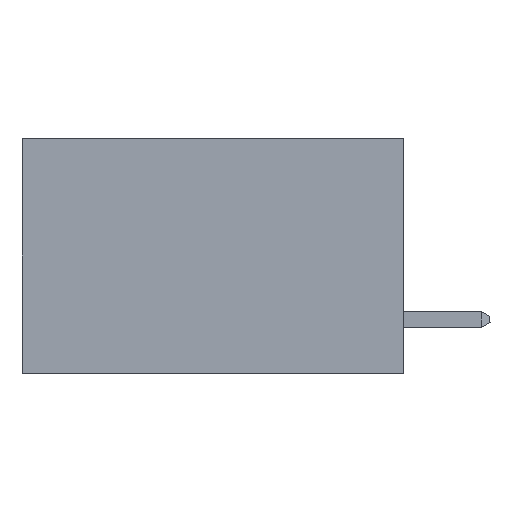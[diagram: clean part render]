
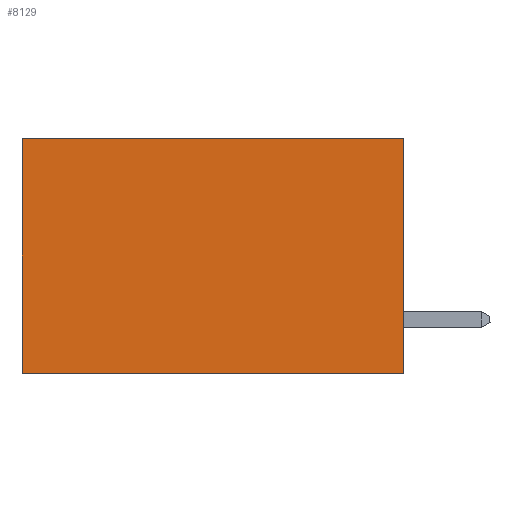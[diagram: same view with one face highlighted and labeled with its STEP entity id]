
A CAD part, left-side view. The second image highlights one B-rep face of the part: STEP entity #8129.
In plain terms, the highlighted planar face has unit normal (-1, 0, 0).
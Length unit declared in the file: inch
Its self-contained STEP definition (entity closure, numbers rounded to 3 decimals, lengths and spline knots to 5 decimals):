
#228 = CARTESIAN_POINT ( 'NONE',  ( 0.2875, 0., 0. ) ) ;
#263 = CARTESIAN_POINT ( 'NONE',  ( 0.2875, 0., 0. ) ) ;
#289 = DIRECTION ( 'NONE',  ( 1., 0., 0. ) ) ;
#298 = CARTESIAN_POINT ( 'NONE',  ( 0.2875, 0.6, 0. ) ) ;
#342 = CARTESIAN_POINT ( 'NONE',  ( 0.2875, 0.6, 0. ) ) ;
#590 = DIRECTION ( 'NONE',  ( 0., 0., -1. ) ) ;
#602 = VECTOR ( 'NONE', #4954, 39.37008 ) ;
#681 = EDGE_CURVE ( 'NONE', #1333, #6982, #4459, .T. ) ;
#813 = ORIENTED_EDGE ( 'NONE', *, *, #3382, .T. ) ;
#1333 = VERTEX_POINT ( 'NONE', #2417 ) ;
#1391 = EDGE_CURVE ( 'NONE', #1656, #2107, #6089, .T. ) ;
#1440 = FACE_OUTER_BOUND ( 'NONE', #5413, .T. ) ;
#1656 = VERTEX_POINT ( 'NONE', #2463 ) ;
#1738 = VECTOR ( 'NONE', #590, 39.37008 ) ;
#1900 = CARTESIAN_POINT ( 'NONE',  ( 0.2875, 0., 0. ) ) ;
#2107 = VERTEX_POINT ( 'NONE', #7534 ) ;
#2406 = EDGE_CURVE ( 'NONE', #1333, #1656, #3311, .T. ) ;
#2417 = CARTESIAN_POINT ( 'NONE',  ( 0.2875, 0., 0. ) ) ;
#2463 = CARTESIAN_POINT ( 'NONE',  ( 0.2875, 0., -0.37 ) ) ;
#2694 = AXIS2_PLACEMENT_3D ( 'NONE', #263, #289, #4822 ) ;
#3311 = LINE ( 'NONE', #1900, #1738 ) ;
#3382 = EDGE_CURVE ( 'NONE', #6982, #2107, #6570, .T. ) ;
#4209 = PLANE ( 'NONE',  #2694 ) ;
#4252 = VECTOR ( 'NONE', #8110, 39.37008 ) ;
#4459 = LINE ( 'NONE', #228, #4252 ) ;
#4574 = DIRECTION ( 'NONE',  ( 0., 1., 0. ) ) ;
#4822 = DIRECTION ( 'NONE',  ( 0., 0., -1. ) ) ;
#4954 = DIRECTION ( 'NONE',  ( 0., 0., -1. ) ) ;
#5007 = ORIENTED_EDGE ( 'NONE', *, *, #681, .T. ) ;
#5413 = EDGE_LOOP ( 'NONE', ( #813, #6239, #6471, #5007 ) ) ;
#6089 = LINE ( 'NONE', #7671, #7725 ) ;
#6239 = ORIENTED_EDGE ( 'NONE', *, *, #1391, .F. ) ;
#6471 = ORIENTED_EDGE ( 'NONE', *, *, #2406, .F. ) ;
#6570 = LINE ( 'NONE', #342, #602 ) ;
#6982 = VERTEX_POINT ( 'NONE', #298 ) ;
#7534 = CARTESIAN_POINT ( 'NONE',  ( 0.2875, 0.6, -0.37 ) ) ;
#7671 = CARTESIAN_POINT ( 'NONE',  ( 0.2875, 0., -0.37 ) ) ;
#7725 = VECTOR ( 'NONE', #4574, 39.37008 ) ;
#8110 = DIRECTION ( 'NONE',  ( 0., 1., 0. ) ) ;
#8129 = ADVANCED_FACE ( 'NONE', ( #1440 ), #4209, .F. ) ;
